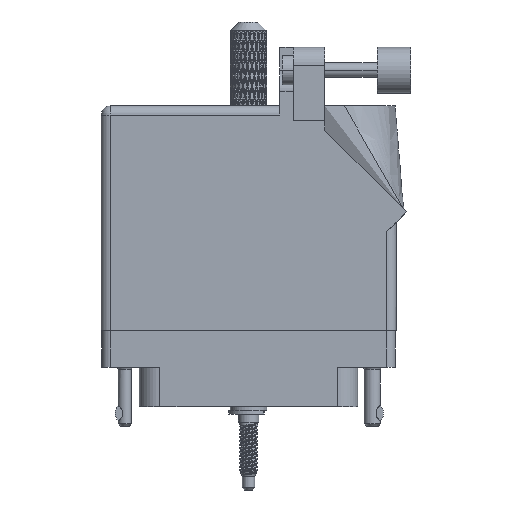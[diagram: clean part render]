
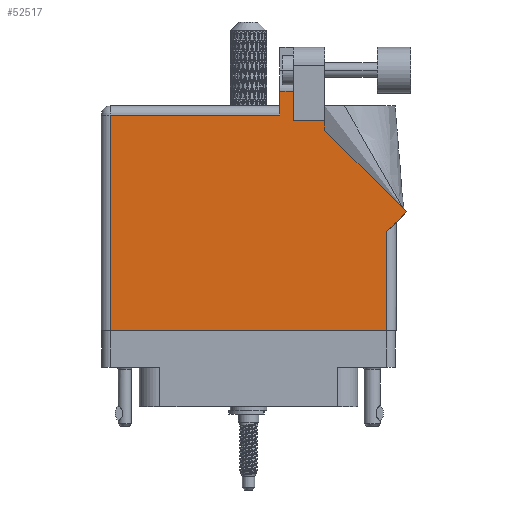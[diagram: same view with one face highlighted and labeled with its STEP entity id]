
A CAD part, front view. The second image highlights one B-rep face of the part: STEP entity #52517.
In plain terms, the highlighted face is planar.
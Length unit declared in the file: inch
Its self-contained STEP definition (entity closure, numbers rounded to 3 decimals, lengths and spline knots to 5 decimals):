
#1642 = VECTOR ( 'NONE', #15410, 39.37008 ) ;
#1796 = VECTOR ( 'NONE', #65757, 39.37008 ) ;
#1853 = LINE ( 'NONE', #85027, #19401 ) ;
#2547 = CARTESIAN_POINT ( 'NONE',  ( -0.943, -0.1, 0.455 ) ) ;
#5009 = ORIENTED_EDGE ( 'NONE', *, *, #63791, .T. ) ;
#5245 = LINE ( 'NONE', #37841, #82067 ) ;
#6265 = DIRECTION ( 'NONE',  ( -1., 0., 0. ) ) ;
#6318 = CARTESIAN_POINT ( 'NONE',  ( -0.943, -0.1, 0.455 ) ) ;
#6663 = CARTESIAN_POINT ( 'NONE',  ( -1.005, -0.1, 0.455 ) ) ;
#8112 = CARTESIAN_POINT ( 'NONE',  ( 0.519, 1.26442, 0.455 ) ) ;
#9789 = VERTEX_POINT ( 'NONE', #76685 ) ;
#10032 = VECTOR ( 'NONE', #79263, 39.37008 ) ;
#10069 = VERTEX_POINT ( 'NONE', #22114 ) ;
#10814 = VECTOR ( 'NONE', #39825, 39.37008 ) ;
#15410 = DIRECTION ( 'NONE',  ( -1., 0., 0. ) ) ;
#16430 = EDGE_CURVE ( 'NONE', #79899, #101499, #88469, .T. ) ;
#17632 = DIRECTION ( 'NONE',  ( -1., 0., 0. ) ) ;
#18782 = EDGE_CURVE ( 'NONE', #22803, #71665, #1853, .T. ) ;
#19401 = VECTOR ( 'NONE', #33848, 39.37008 ) ;
#22114 = CARTESIAN_POINT ( 'NONE',  ( 0.943, -0.1, 0.455 ) ) ;
#22803 = VERTEX_POINT ( 'NONE', #43413 ) ;
#23812 = VECTOR ( 'NONE', #100384, 39.37008 ) ;
#24576 = LINE ( 'NONE', #66902, #1642 ) ;
#24673 = CARTESIAN_POINT ( 'NONE',  ( 0.212, 1.5315, 0.455 ) ) ;
#25795 = EDGE_CURVE ( 'NONE', #101499, #90785, #100692, .T. ) ;
#26420 = ORIENTED_EDGE ( 'NONE', *, *, #25795, .T. ) ;
#26703 = FACE_OUTER_BOUND ( 'NONE', #100009, .T. ) ;
#26905 = DIRECTION ( 'NONE',  ( 0., 1., 0. ) ) ;
#28490 = LINE ( 'NONE', #53472, #29897 ) ;
#29897 = VECTOR ( 'NONE', #105382, 39.37008 ) ;
#30389 = EDGE_CURVE ( 'NONE', #91358, #79899, #28490, .T. ) ;
#31624 = CARTESIAN_POINT ( 'NONE',  ( -1.005, 1.368, 0.455 ) ) ;
#33458 = ORIENTED_EDGE ( 'NONE', *, *, #105634, .T. ) ;
#33848 = DIRECTION ( 'NONE',  ( 0.707, 0.707, 0. ) ) ;
#36278 = ORIENTED_EDGE ( 'NONE', *, *, #104400, .T. ) ;
#37841 = CARTESIAN_POINT ( 'NONE',  ( 1.07571, 0.70771, 0.455 ) ) ;
#39101 = VERTEX_POINT ( 'NONE', #8112 ) ;
#39825 = DIRECTION ( 'NONE',  ( 0., 1., 0. ) ) ;
#43413 = CARTESIAN_POINT ( 'NONE',  ( 0.943, 0.575, 0.455 ) ) ;
#44169 = VECTOR ( 'NONE', #26905, 39.37008 ) ;
#44358 = DIRECTION ( 'NONE',  ( 0., -1., 0. ) ) ;
#45007 = CARTESIAN_POINT ( 'NONE',  ( 0.63677, 1.5315, 0.455 ) ) ;
#45212 = EDGE_CURVE ( 'NONE', #90785, #10069, #86690, .T. ) ;
#45924 = ORIENTED_EDGE ( 'NONE', *, *, #16430, .T. ) ;
#47655 = ORIENTED_EDGE ( 'NONE', *, *, #86436, .T. ) ;
#51186 = CARTESIAN_POINT ( 'NONE',  ( 0.306, 1.33, 0.455 ) ) ;
#52517 = ADVANCED_FACE ( 'NONE', ( #26703 ), #58532, .F. ) ;
#52886 = CARTESIAN_POINT ( 'NONE',  ( 0.943, 0.637, 0.455 ) ) ;
#53472 = CARTESIAN_POINT ( 'NONE',  ( 0.212, 1.43, 0.455 ) ) ;
#53776 = VERTEX_POINT ( 'NONE', #84609 ) ;
#54176 = CARTESIAN_POINT ( 'NONE',  ( 1.07571, 0.70771, 0.455 ) ) ;
#58532 = PLANE ( 'NONE',  #82294 ) ;
#60447 = ORIENTED_EDGE ( 'NONE', *, *, #18782, .T. ) ;
#62451 = ORIENTED_EDGE ( 'NONE', *, *, #45212, .T. ) ;
#63791 = EDGE_CURVE ( 'NONE', #100216, #53776, #86210, .T. ) ;
#65757 = DIRECTION ( 'NONE',  ( 1., 0., 0. ) ) ;
#66902 = CARTESIAN_POINT ( 'NONE',  ( 0.519, 1.33, 0.455 ) ) ;
#67687 = ORIENTED_EDGE ( 'NONE', *, *, #88786, .T. ) ;
#71665 = VERTEX_POINT ( 'NONE', #54176 ) ;
#74398 = CARTESIAN_POINT ( 'NONE',  ( 0.306, 1.33, 0.455 ) ) ;
#76223 = CARTESIAN_POINT ( 'NONE',  ( -1.005, 1.43, 0.455 ) ) ;
#76685 = CARTESIAN_POINT ( 'NONE',  ( 0.519, 1.33, 0.455 ) ) ;
#77847 = VECTOR ( 'NONE', #44358, 39.37008 ) ;
#78000 = CARTESIAN_POINT ( 'NONE',  ( 0.519, 1.26442, 0.455 ) ) ;
#79263 = DIRECTION ( 'NONE',  ( 0., 1., 0. ) ) ;
#79899 = VERTEX_POINT ( 'NONE', #95636 ) ;
#81426 = LINE ( 'NONE', #52886, #10032 ) ;
#82067 = VECTOR ( 'NONE', #97914, 39.37008 ) ;
#82294 = AXIS2_PLACEMENT_3D ( 'NONE', #76223, #93170, #6265 ) ;
#84609 = CARTESIAN_POINT ( 'NONE',  ( 0.306, 1.5315, 0.455 ) ) ;
#85027 = CARTESIAN_POINT ( 'NONE',  ( 1.005, 0.637, 0.455 ) ) ;
#86210 = LINE ( 'NONE', #74398, #10814 ) ;
#86436 = EDGE_CURVE ( 'NONE', #10069, #22803, #81426, .T. ) ;
#86690 = LINE ( 'NONE', #6663, #1796 ) ;
#88469 = LINE ( 'NONE', #31624, #23812 ) ;
#88786 = EDGE_CURVE ( 'NONE', #9789, #100216, #24576, .T. ) ;
#90785 = VERTEX_POINT ( 'NONE', #6318 ) ;
#91064 = ORIENTED_EDGE ( 'NONE', *, *, #30389, .T. ) ;
#91358 = VERTEX_POINT ( 'NONE', #24673 ) ;
#93170 = DIRECTION ( 'NONE',  ( 0., 0., -1. ) ) ;
#95636 = CARTESIAN_POINT ( 'NONE',  ( 0.212, 1.368, 0.455 ) ) ;
#96176 = ORIENTED_EDGE ( 'NONE', *, *, #98649, .T. ) ;
#97914 = DIRECTION ( 'NONE',  ( -0.707, 0.707, 0. ) ) ;
#98649 = EDGE_CURVE ( 'NONE', #53776, #91358, #109432, .T. ) ;
#100009 = EDGE_LOOP ( 'NONE', ( #5009, #96176, #91064, #45924, #26420, #62451, #47655, #60447, #36278, #33458, #67687 ) ) ;
#100216 = VERTEX_POINT ( 'NONE', #51186 ) ;
#100384 = DIRECTION ( 'NONE',  ( -1., 0., 0. ) ) ;
#100692 = LINE ( 'NONE', #2547, #77847 ) ;
#101499 = VERTEX_POINT ( 'NONE', #105489 ) ;
#103407 = LINE ( 'NONE', #78000, #44169 ) ;
#104400 = EDGE_CURVE ( 'NONE', #71665, #39101, #5245, .T. ) ;
#105382 = DIRECTION ( 'NONE',  ( 0., -1., 0. ) ) ;
#105489 = CARTESIAN_POINT ( 'NONE',  ( -0.943, 1.368, 0.455 ) ) ;
#105634 = EDGE_CURVE ( 'NONE', #39101, #9789, #103407, .T. ) ;
#106882 = VECTOR ( 'NONE', #17632, 39.37008 ) ;
#109432 = LINE ( 'NONE', #45007, #106882 ) ;
